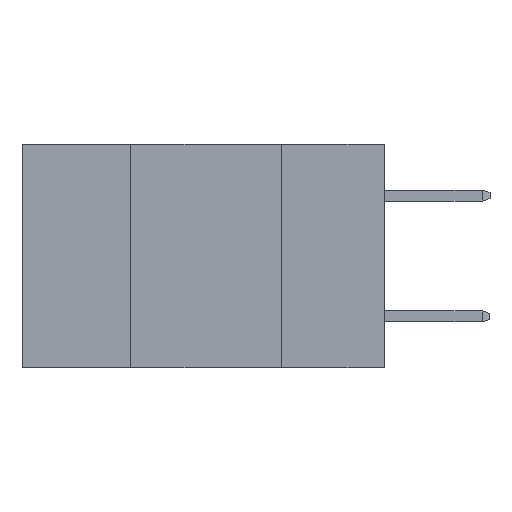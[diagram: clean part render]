
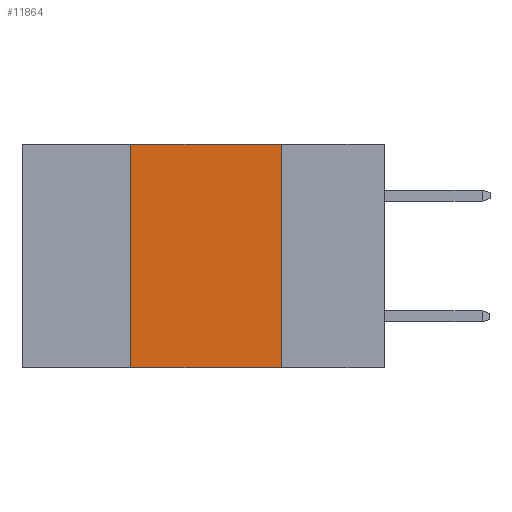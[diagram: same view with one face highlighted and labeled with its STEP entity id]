
A CAD part, left-side view. The second image highlights one B-rep face of the part: STEP entity #11864.
In plain terms, the highlighted planar face has unit normal (-1, 0, 0).
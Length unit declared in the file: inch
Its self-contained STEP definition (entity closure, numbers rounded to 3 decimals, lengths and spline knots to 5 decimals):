
#1864 = CARTESIAN_POINT ( 'NONE',  ( 0., 0.17, -0.37 ) ) ;
#2068 = DIRECTION ( 'NONE',  ( 0., 0., 1. ) ) ;
#2088 = FACE_OUTER_BOUND ( 'NONE', #2361, .T. ) ;
#2168 = CARTESIAN_POINT ( 'NONE',  ( 0., 0.17, 0. ) ) ;
#2361 = EDGE_LOOP ( 'NONE', ( #10169, #10180, #10272, #10341 ) ) ;
#2997 = DIRECTION ( 'NONE',  ( 1., 0., 0. ) ) ;
#3058 = EDGE_CURVE ( 'NONE', #10630, #11708, #3904, .T. ) ;
#3651 = LINE ( 'NONE', #9218, #8514 ) ;
#3904 = LINE ( 'NONE', #7886, #4224 ) ;
#4224 = VECTOR ( 'NONE', #2068, 39.37008 ) ;
#4355 = CARTESIAN_POINT ( 'NONE',  ( 0., 0.17, 0. ) ) ;
#4921 = PLANE ( 'NONE',  #6416 ) ;
#5413 = DIRECTION ( 'NONE',  ( 0., -1., 0. ) ) ;
#5723 = CARTESIAN_POINT ( 'NONE',  ( 0., 0.6, -0.37 ) ) ;
#5765 = VECTOR ( 'NONE', #10122, 39.37008 ) ;
#5771 = CARTESIAN_POINT ( 'NONE',  ( 0., 0.42, 0. ) ) ;
#5926 = VECTOR ( 'NONE', #6722, 39.37008 ) ;
#6416 = AXIS2_PLACEMENT_3D ( 'NONE', #8803, #2997, #9745 ) ;
#6722 = DIRECTION ( 'NONE',  ( 0., -1., 0. ) ) ;
#7641 = EDGE_CURVE ( 'NONE', #11708, #11988, #3651, .T. ) ;
#7711 = LINE ( 'NONE', #4355, #5765 ) ;
#7886 = CARTESIAN_POINT ( 'NONE',  ( 0., 0.42, 0. ) ) ;
#8514 = VECTOR ( 'NONE', #5413, 39.37008 ) ;
#8803 = CARTESIAN_POINT ( 'NONE',  ( 0., 0.6, 0. ) ) ;
#9218 = CARTESIAN_POINT ( 'NONE',  ( 0., 0.6, 0. ) ) ;
#9745 = DIRECTION ( 'NONE',  ( 0., 0., -1. ) ) ;
#10101 = VERTEX_POINT ( 'NONE', #1864 ) ;
#10122 = DIRECTION ( 'NONE',  ( 0., 0., -1. ) ) ;
#10169 = ORIENTED_EDGE ( 'NONE', *, *, #12242, .F. ) ;
#10180 = ORIENTED_EDGE ( 'NONE', *, *, #7641, .F. ) ;
#10272 = ORIENTED_EDGE ( 'NONE', *, *, #3058, .F. ) ;
#10341 = ORIENTED_EDGE ( 'NONE', *, *, #11638, .T. ) ;
#10630 = VERTEX_POINT ( 'NONE', #12033 ) ;
#10941 = LINE ( 'NONE', #5723, #5926 ) ;
#11638 = EDGE_CURVE ( 'NONE', #10630, #10101, #10941, .T. ) ;
#11708 = VERTEX_POINT ( 'NONE', #5771 ) ;
#11864 = ADVANCED_FACE ( 'NONE', ( #2088 ), #4921, .F. ) ;
#11988 = VERTEX_POINT ( 'NONE', #2168 ) ;
#12033 = CARTESIAN_POINT ( 'NONE',  ( 0., 0.42, -0.37 ) ) ;
#12242 = EDGE_CURVE ( 'NONE', #11988, #10101, #7711, .T. ) ;
